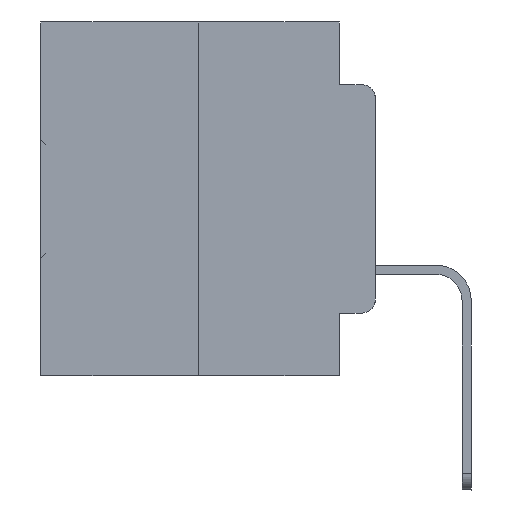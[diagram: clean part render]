
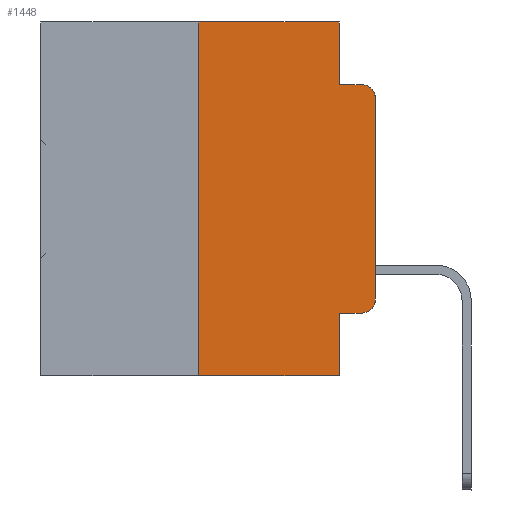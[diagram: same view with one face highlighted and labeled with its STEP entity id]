
A CAD part, left-side view. The second image highlights one B-rep face of the part: STEP entity #1448.
In plain terms, the highlighted planar face has unit normal (-1, 0, 0).
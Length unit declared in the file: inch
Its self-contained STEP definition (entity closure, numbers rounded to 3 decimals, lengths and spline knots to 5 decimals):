
#676 = ORIENTED_EDGE ( 'NONE', *, *, #25888, .T. ) ;
#867 = LINE ( 'NONE', #10989, #2109 ) ;
#1275 = CARTESIAN_POINT ( 'NONE',  ( 0., 0.051, -0.0885 ) ) ;
#1426 = CARTESIAN_POINT ( 'NONE',  ( 0., 0.25, 0. ) ) ;
#1448 = ADVANCED_FACE ( 'NONE', ( #25699 ), #24234, .F. ) ;
#1529 = DIRECTION ( 'NONE',  ( 0., -1., 0. ) ) ;
#1532 = CARTESIAN_POINT ( 'NONE',  ( 0., 0., -0.1085 ) ) ;
#2109 = VECTOR ( 'NONE', #15966, 39.37008 ) ;
#2193 = EDGE_CURVE ( 'NONE', #25026, #13778, #11414, .T. ) ;
#2253 = CARTESIAN_POINT ( 'NONE',  ( 0., 0.051, -0.0885 ) ) ;
#2519 = LINE ( 'NONE', #1275, #15495 ) ;
#2594 = EDGE_CURVE ( 'NONE', #9368, #18516, #22585, .T. ) ;
#2980 = VECTOR ( 'NONE', #31649, 39.37008 ) ;
#3596 = DIRECTION ( 'NONE',  ( 0., 0., -1. ) ) ;
#3616 = LINE ( 'NONE', #9757, #21875 ) ;
#3784 = CARTESIAN_POINT ( 'NONE',  ( 0., 0.02, -0.1085 ) ) ;
#3816 = CARTESIAN_POINT ( 'NONE',  ( 0., 0.051, -0.4115 ) ) ;
#3912 = ORIENTED_EDGE ( 'NONE', *, *, #21572, .T. ) ;
#4061 = VERTEX_POINT ( 'NONE', #31146 ) ;
#4552 = VECTOR ( 'NONE', #14541, 39.37008 ) ;
#4989 = EDGE_CURVE ( 'NONE', #16012, #13778, #2519, .T. ) ;
#5038 = EDGE_CURVE ( 'NONE', #25059, #8660, #28497, .T. ) ;
#6342 = VECTOR ( 'NONE', #1529, 39.37008 ) ;
#6588 = CARTESIAN_POINT ( 'NONE',  ( 0., 0.02, -0.0885 ) ) ;
#6618 = CARTESIAN_POINT ( 'NONE',  ( 0., 0.473, 0. ) ) ;
#6755 = VECTOR ( 'NONE', #23361, 39.37008 ) ;
#7179 = VECTOR ( 'NONE', #16431, 39.37008 ) ;
#7215 = EDGE_CURVE ( 'NONE', #8660, #16012, #9205, .T. ) ;
#7443 = DIRECTION ( 'NONE',  ( 0., 0., -1. ) ) ;
#8660 = VERTEX_POINT ( 'NONE', #12346 ) ;
#8706 = CARTESIAN_POINT ( 'NONE',  ( 0., 0.473, 0. ) ) ;
#9076 = CARTESIAN_POINT ( 'NONE',  ( 0., 0.25, -0.5 ) ) ;
#9205 = LINE ( 'NONE', #12590, #6755 ) ;
#9368 = VERTEX_POINT ( 'NONE', #13082 ) ;
#9757 = CARTESIAN_POINT ( 'NONE',  ( 0., 0.25, 0. ) ) ;
#9821 = CARTESIAN_POINT ( 'NONE',  ( 0., 0.02, -0.3915 ) ) ;
#10925 = CARTESIAN_POINT ( 'NONE',  ( 0., 0.051, 0. ) ) ;
#10989 = CARTESIAN_POINT ( 'NONE',  ( 0., 0., 0. ) ) ;
#11246 = LINE ( 'NONE', #29030, #7179 ) ;
#11314 = DIRECTION ( 'NONE',  ( 1., 0., 0. ) ) ;
#11414 = CIRCLE ( 'NONE', #16510, 0.02 ) ;
#12069 = ORIENTED_EDGE ( 'NONE', *, *, #4989, .F. ) ;
#12108 = VERTEX_POINT ( 'NONE', #9076 ) ;
#12319 = LINE ( 'NONE', #10925, #2980 ) ;
#12346 = CARTESIAN_POINT ( 'NONE',  ( 0., 0.051, 0. ) ) ;
#12590 = CARTESIAN_POINT ( 'NONE',  ( 0., 0.051, 0. ) ) ;
#13082 = CARTESIAN_POINT ( 'NONE',  ( 0., 0.051, -0.4115 ) ) ;
#13778 = VERTEX_POINT ( 'NONE', #6588 ) ;
#13830 = ORIENTED_EDGE ( 'NONE', *, *, #2193, .T. ) ;
#13855 = ORIENTED_EDGE ( 'NONE', *, *, #2594, .T. ) ;
#14355 = CARTESIAN_POINT ( 'NONE',  ( 0., 0.02, -0.4115 ) ) ;
#14541 = DIRECTION ( 'NONE',  ( 0., -1., 0. ) ) ;
#14626 = DIRECTION ( 'NONE',  ( 0., 0., 1. ) ) ;
#14742 = ORIENTED_EDGE ( 'NONE', *, *, #28811, .T. ) ;
#14826 = AXIS2_PLACEMENT_3D ( 'NONE', #9821, #28291, #7443 ) ;
#15495 = VECTOR ( 'NONE', #19542, 39.37008 ) ;
#15624 = AXIS2_PLACEMENT_3D ( 'NONE', #8706, #11314, #3596 ) ;
#15966 = DIRECTION ( 'NONE',  ( 0., 0., 1. ) ) ;
#16012 = VERTEX_POINT ( 'NONE', #2253 ) ;
#16431 = DIRECTION ( 'NONE',  ( 0., -1., 0. ) ) ;
#16510 = AXIS2_PLACEMENT_3D ( 'NONE', #3784, #27488, #19545 ) ;
#16780 = CIRCLE ( 'NONE', #14826, 0.02 ) ;
#18006 = ORIENTED_EDGE ( 'NONE', *, *, #5038, .F. ) ;
#18114 = CARTESIAN_POINT ( 'NONE',  ( 0., 0.051, -0.5 ) ) ;
#18516 = VERTEX_POINT ( 'NONE', #14355 ) ;
#18591 = EDGE_LOOP ( 'NONE', ( #14742, #13830, #12069, #26665, #18006, #32682, #676, #24029, #13855, #3912 ) ) ;
#19542 = DIRECTION ( 'NONE',  ( 0., -1., 0. ) ) ;
#19545 = DIRECTION ( 'NONE',  ( 0., 0., -1. ) ) ;
#19748 = EDGE_CURVE ( 'NONE', #12108, #25059, #3616, .T. ) ;
#21572 = EDGE_CURVE ( 'NONE', #18516, #4061, #16780, .T. ) ;
#21875 = VECTOR ( 'NONE', #14626, 39.37008 ) ;
#22585 = LINE ( 'NONE', #3816, #6342 ) ;
#23361 = DIRECTION ( 'NONE',  ( 0., 0., -1. ) ) ;
#24029 = ORIENTED_EDGE ( 'NONE', *, *, #30759, .F. ) ;
#24234 = PLANE ( 'NONE',  #15624 ) ;
#25026 = VERTEX_POINT ( 'NONE', #1532 ) ;
#25059 = VERTEX_POINT ( 'NONE', #1426 ) ;
#25699 = FACE_OUTER_BOUND ( 'NONE', #18591, .T. ) ;
#25888 = EDGE_CURVE ( 'NONE', #12108, #27160, #11246, .T. ) ;
#26665 = ORIENTED_EDGE ( 'NONE', *, *, #7215, .F. ) ;
#27160 = VERTEX_POINT ( 'NONE', #18114 ) ;
#27488 = DIRECTION ( 'NONE',  ( -1., 0., 0. ) ) ;
#28291 = DIRECTION ( 'NONE',  ( -1., 0., 0. ) ) ;
#28497 = LINE ( 'NONE', #6618, #4552 ) ;
#28811 = EDGE_CURVE ( 'NONE', #4061, #25026, #867, .T. ) ;
#29030 = CARTESIAN_POINT ( 'NONE',  ( 0., 0.473, -0.5 ) ) ;
#30759 = EDGE_CURVE ( 'NONE', #9368, #27160, #12319, .T. ) ;
#31146 = CARTESIAN_POINT ( 'NONE',  ( 0., 0., -0.3915 ) ) ;
#31649 = DIRECTION ( 'NONE',  ( 0., 0., -1. ) ) ;
#32682 = ORIENTED_EDGE ( 'NONE', *, *, #19748, .F. ) ;
